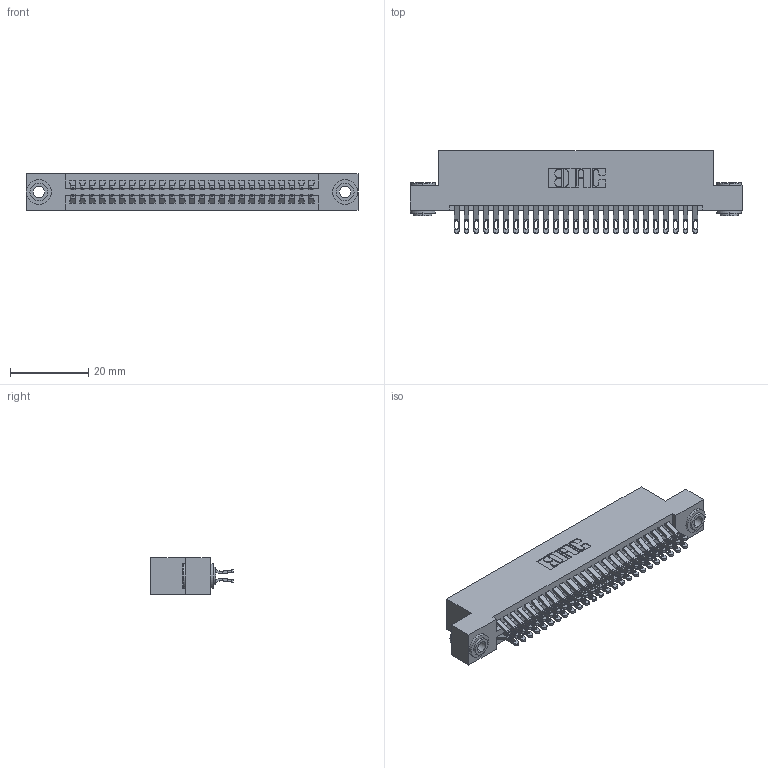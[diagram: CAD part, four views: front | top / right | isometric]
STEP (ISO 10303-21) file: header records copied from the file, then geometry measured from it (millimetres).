
FILE_DESCRIPTION (( 'STEP AP203' ), '1' );
FILE_NAME ('395-050-555-203.STEP', '2019-10-19T13:53:28', ( '' ), ( '' ), 'SwSTEP 2.0', 'SolidWorks 2016', '' );
FILE_SCHEMA (( 'CONFIG_CONTROL_DESIGN' ));
Length unit declared in the file: inch
Products named in the file (4): 395-050-555-203; 345 Part_Flush Mounting Lugs - 0.156 Dia-TH; 345-292-001_555 Tail; 345-250-002_345-250-002-102
Assembly tree (53 placements, depth 2):
  395-050-555-203
    345 Part_Flush Mounting Lugs - 0.156 Dia-TH
    345-292-001_555 Tail  x50
    345-250-002_345-250-002-102  x2
Bounding box: 84.71 x 21.13 x 9.4 mm (x, y, z)
Volume: 8235.3 mm3; surface area: 12553.3 mm2
Topology: 53 solids, 53 shells, 2964 faces, 9267 edges, 6174 vertices
Faces by surface type: plane 1640, cylinder 1316, cone 8
Entity records: 22880 total; most frequent: CARTESIAN_POINT 3861, ORIENTED_EDGE 3758, DIRECTION 3425, EDGE_CURVE 1879, VECTOR 1603, LINE 1603, VERTEX_POINT 1250, AXIS2_PLACEMENT_3D 911
